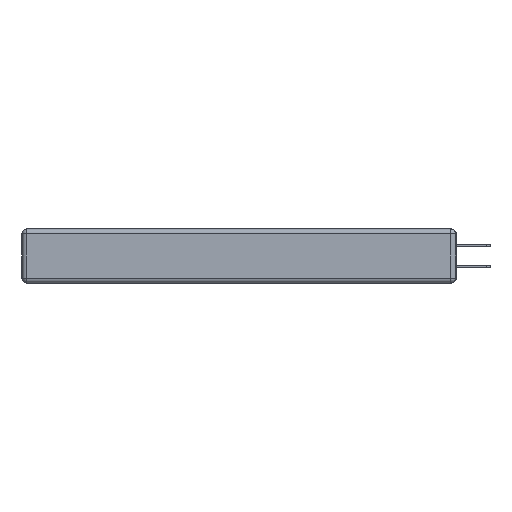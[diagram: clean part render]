
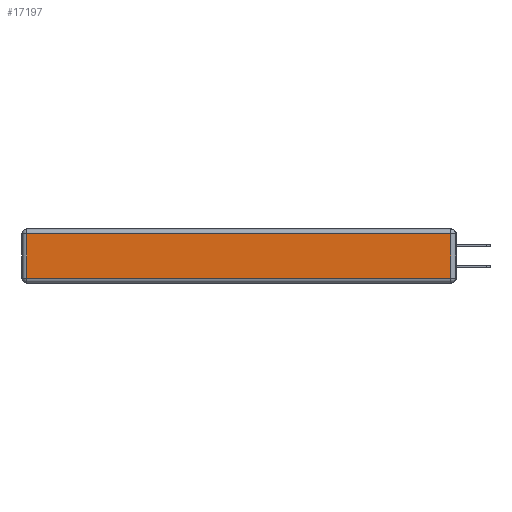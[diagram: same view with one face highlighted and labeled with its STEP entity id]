
A CAD part, left-side view. The second image highlights one B-rep face of the part: STEP entity #17197.
In plain terms, the highlighted planar face has unit normal (-1, 0, 0).
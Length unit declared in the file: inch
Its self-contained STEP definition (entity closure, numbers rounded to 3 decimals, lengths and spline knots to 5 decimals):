
#415 = ORIENTED_EDGE ( 'NONE', *, *, #13912, .T. ) ;
#523 = CARTESIAN_POINT ( 'NONE',  ( 0., 2.75, -0.03 ) ) ;
#1669 = VECTOR ( 'NONE', #5907, 39.37008 ) ;
#2022 = EDGE_CURVE ( 'NONE', #15472, #17015, #10311, .T. ) ;
#2463 = EDGE_LOOP ( 'NONE', ( #8589, #19109, #4775, #415 ) ) ;
#2553 = DIRECTION ( 'NONE',  ( 0., 1., 0. ) ) ;
#4356 = CARTESIAN_POINT ( 'NONE',  ( 0., 0., -0.313 ) ) ;
#4477 = CARTESIAN_POINT ( 'NONE',  ( 0., 0.03, -0.03 ) ) ;
#4775 = ORIENTED_EDGE ( 'NONE', *, *, #11246, .T. ) ;
#4788 = CARTESIAN_POINT ( 'NONE',  ( 0., 0.03, -0.343 ) ) ;
#4862 = CARTESIAN_POINT ( 'NONE',  ( 0., 2.72, -0.03 ) ) ;
#5206 = VECTOR ( 'NONE', #6817, 39.37008 ) ;
#5907 = DIRECTION ( 'NONE',  ( 0., -1., 0. ) ) ;
#6375 = DIRECTION ( 'NONE',  ( 0., 0., 1. ) ) ;
#6817 = DIRECTION ( 'NONE',  ( 0., 0., 1. ) ) ;
#7724 = CARTESIAN_POINT ( 'NONE',  ( 0., 0., -0.343 ) ) ;
#8589 = ORIENTED_EDGE ( 'NONE', *, *, #17381, .T. ) ;
#8915 = LINE ( 'NONE', #523, #14453 ) ;
#10311 = LINE ( 'NONE', #4788, #5206 ) ;
#11246 = EDGE_CURVE ( 'NONE', #17015, #19921, #8915, .T. ) ;
#13443 = FACE_OUTER_BOUND ( 'NONE', #2463, .T. ) ;
#13912 = EDGE_CURVE ( 'NONE', #19921, #21191, #22152, .T. ) ;
#14453 = VECTOR ( 'NONE', #2553, 39.37008 ) ;
#14556 = PLANE ( 'NONE',  #20087 ) ;
#14632 = CARTESIAN_POINT ( 'NONE',  ( 0., 0.03, -0.313 ) ) ;
#15056 = LINE ( 'NONE', #4356, #1669 ) ;
#15472 = VERTEX_POINT ( 'NONE', #14632 ) ;
#17015 = VERTEX_POINT ( 'NONE', #4477 ) ;
#17197 = ADVANCED_FACE ( 'NONE', ( #13443 ), #14556, .T. ) ;
#17381 = EDGE_CURVE ( 'NONE', #21191, #15472, #15056, .T. ) ;
#18036 = CARTESIAN_POINT ( 'NONE',  ( 0., 2.72, -0.313 ) ) ;
#18498 = DIRECTION ( 'NONE',  ( -1., 0., 0. ) ) ;
#18665 = VECTOR ( 'NONE', #21912, 39.37008 ) ;
#19109 = ORIENTED_EDGE ( 'NONE', *, *, #2022, .T. ) ;
#19921 = VERTEX_POINT ( 'NONE', #4862 ) ;
#20087 = AXIS2_PLACEMENT_3D ( 'NONE', #7724, #18498, #6375 ) ;
#20331 = CARTESIAN_POINT ( 'NONE',  ( 0., 2.72, -0.343 ) ) ;
#21191 = VERTEX_POINT ( 'NONE', #18036 ) ;
#21912 = DIRECTION ( 'NONE',  ( 0., 0., -1. ) ) ;
#22152 = LINE ( 'NONE', #20331, #18665 ) ;
